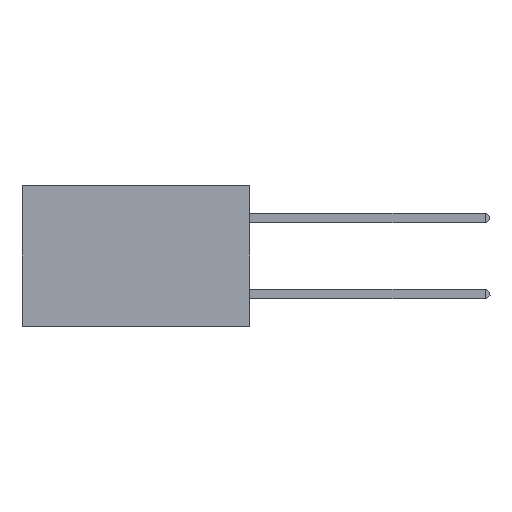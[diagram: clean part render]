
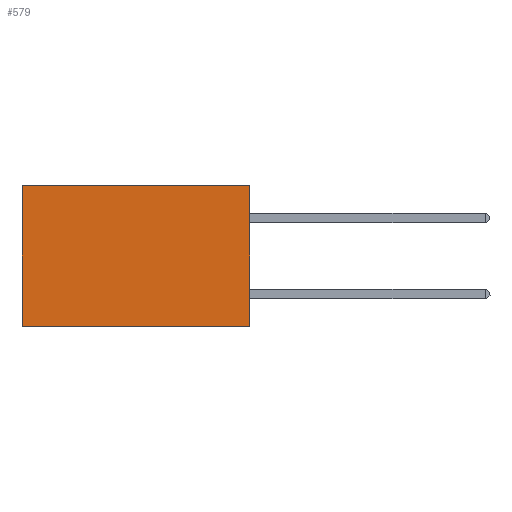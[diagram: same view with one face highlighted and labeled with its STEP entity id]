
A CAD part, left-side view. The second image highlights one B-rep face of the part: STEP entity #579.
In plain terms, the highlighted planar face has unit normal (-1, 0, 0).
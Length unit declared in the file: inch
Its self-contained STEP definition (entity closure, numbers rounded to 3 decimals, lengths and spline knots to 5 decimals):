
#429 = ORIENTED_EDGE ( 'NONE', *, *, #2439, .T. ) ;
#579 = ADVANCED_FACE ( 'NONE', ( #4497 ), #11261, .F. ) ;
#709 = DIRECTION ( 'NONE',  ( 0., 0., -1. ) ) ;
#994 = CARTESIAN_POINT ( 'NONE',  ( 0.2875, 0., 0. ) ) ;
#1686 = CARTESIAN_POINT ( 'NONE',  ( 0.2875, 0., 0. ) ) ;
#1841 = DIRECTION ( 'NONE',  ( 0., 1., 0. ) ) ;
#1935 = VERTEX_POINT ( 'NONE', #1686 ) ;
#2149 = CARTESIAN_POINT ( 'NONE',  ( 0.2875, 0.6, -0.37 ) ) ;
#2204 = VERTEX_POINT ( 'NONE', #4104 ) ;
#2401 = DIRECTION ( 'NONE',  ( 0., 1., 0. ) ) ;
#2439 = EDGE_CURVE ( 'NONE', #1935, #2204, #5257, .T. ) ;
#2476 = CARTESIAN_POINT ( 'NONE',  ( 0.2875, 0., -0.37 ) ) ;
#3639 = EDGE_CURVE ( 'NONE', #1935, #10609, #6581, .T. ) ;
#3904 = EDGE_CURVE ( 'NONE', #10609, #4643, #10231, .T. ) ;
#4023 = CARTESIAN_POINT ( 'NONE',  ( 0.2875, 0., -0.37 ) ) ;
#4078 = ORIENTED_EDGE ( 'NONE', *, *, #3904, .F. ) ;
#4104 = CARTESIAN_POINT ( 'NONE',  ( 0.2875, 0.6, 0. ) ) ;
#4497 = FACE_OUTER_BOUND ( 'NONE', #8748, .T. ) ;
#4643 = VERTEX_POINT ( 'NONE', #2149 ) ;
#4966 = EDGE_CURVE ( 'NONE', #2204, #4643, #9512, .T. ) ;
#5257 = LINE ( 'NONE', #994, #9998 ) ;
#5795 = ORIENTED_EDGE ( 'NONE', *, *, #4966, .T. ) ;
#6192 = CARTESIAN_POINT ( 'NONE',  ( 0.2875, 0., 0. ) ) ;
#6581 = LINE ( 'NONE', #6192, #9412 ) ;
#7032 = DIRECTION ( 'NONE',  ( 0., 0., -1. ) ) ;
#7094 = ORIENTED_EDGE ( 'NONE', *, *, #3639, .F. ) ;
#7840 = DIRECTION ( 'NONE',  ( 0., 0., -1. ) ) ;
#8076 = CARTESIAN_POINT ( 'NONE',  ( 0.2875, 0., 0. ) ) ;
#8748 = EDGE_LOOP ( 'NONE', ( #5795, #4078, #7094, #429 ) ) ;
#8923 = AXIS2_PLACEMENT_3D ( 'NONE', #8076, #10369, #7840 ) ;
#9412 = VECTOR ( 'NONE', #7032, 39.37008 ) ;
#9414 = CARTESIAN_POINT ( 'NONE',  ( 0.2875, 0.6, 0. ) ) ;
#9512 = LINE ( 'NONE', #9414, #11175 ) ;
#9998 = VECTOR ( 'NONE', #1841, 39.37008 ) ;
#10231 = LINE ( 'NONE', #2476, #11202 ) ;
#10369 = DIRECTION ( 'NONE',  ( 1., 0., 0. ) ) ;
#10609 = VERTEX_POINT ( 'NONE', #4023 ) ;
#11175 = VECTOR ( 'NONE', #709, 39.37008 ) ;
#11202 = VECTOR ( 'NONE', #2401, 39.37008 ) ;
#11261 = PLANE ( 'NONE',  #8923 ) ;
